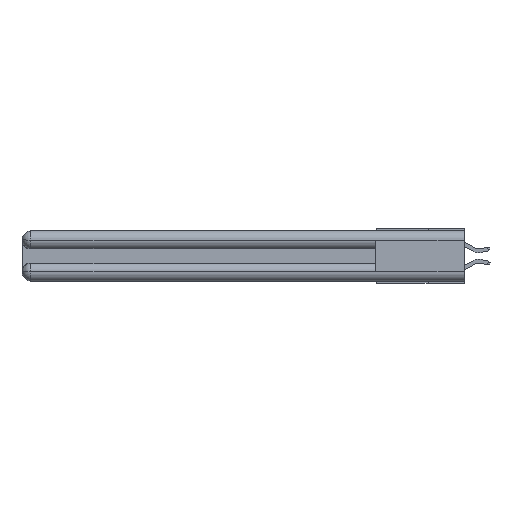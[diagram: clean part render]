
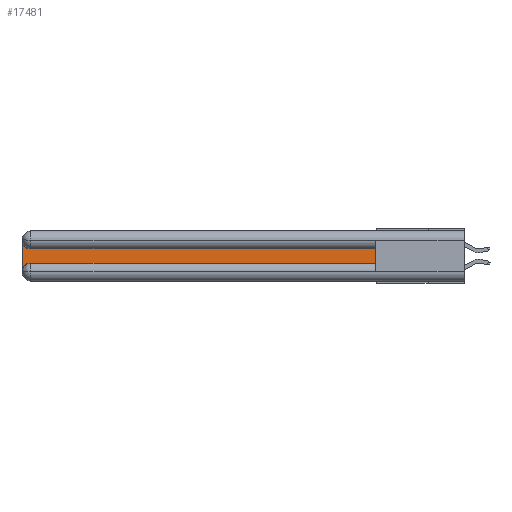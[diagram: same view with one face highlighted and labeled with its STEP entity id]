
A CAD part, left-side view. The second image highlights one B-rep face of the part: STEP entity #17481.
In plain terms, the highlighted planar face has unit normal (-1, 0, 0).
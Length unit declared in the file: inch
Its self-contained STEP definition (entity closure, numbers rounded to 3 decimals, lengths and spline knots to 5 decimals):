
#109 = AXIS2_PLACEMENT_3D ( 'NONE', #12864, #20478, #27432 ) ;
#374 = EDGE_CURVE ( 'NONE', #18083, #17569, #11368, .T. ) ;
#1002 = EDGE_LOOP ( 'NONE', ( #25631, #18869, #18796, #18351, #6841, #10107 ) ) ;
#1328 = CARTESIAN_POINT ( 'NONE',  ( 0.075, 3., -0.0625 ) ) ;
#2735 = EDGE_CURVE ( 'NONE', #17606, #11998, #6616, .T. ) ;
#4103 = DIRECTION ( 'NONE',  ( 0., 0., -1. ) ) ;
#4303 = LINE ( 'NONE', #16576, #23437 ) ;
#5975 = VERTEX_POINT ( 'NONE', #31462 ) ;
#6616 = LINE ( 'NONE', #9238, #14038 ) ;
#6841 = ORIENTED_EDGE ( 'NONE', *, *, #374, .T. ) ;
#8854 = DIRECTION ( 'NONE',  ( 0., 1., 0. ) ) ;
#8981 = EDGE_CURVE ( 'NONE', #17569, #5975, #31895, .T. ) ;
#9238 = CARTESIAN_POINT ( 'NONE',  ( 0.075, 3., -0.2175 ) ) ;
#10107 = ORIENTED_EDGE ( 'NONE', *, *, #8981, .T. ) ;
#11368 = LINE ( 'NONE', #29456, #12926 ) ;
#11998 = VERTEX_POINT ( 'NONE', #20435 ) ;
#12864 = CARTESIAN_POINT ( 'NONE',  ( 0.075, 2.94, -0.0625 ) ) ;
#12926 = VECTOR ( 'NONE', #17162, 39.37008 ) ;
#14038 = VECTOR ( 'NONE', #4103, 39.37008 ) ;
#15413 = DIRECTION ( 'NONE',  ( 0., 0., -1. ) ) ;
#16024 = AXIS2_PLACEMENT_3D ( 'NONE', #31465, #26398, #19001 ) ;
#16123 = CARTESIAN_POINT ( 'NONE',  ( 0.075, 2.94, -0.2175 ) ) ;
#16141 = VERTEX_POINT ( 'NONE', #28386 ) ;
#16576 = CARTESIAN_POINT ( 'NONE',  ( 0.075, 0.6, -0.1225 ) ) ;
#17162 = DIRECTION ( 'NONE',  ( 0., -1., 0. ) ) ;
#17481 = ADVANCED_FACE ( 'NONE', ( #19691 ), #20323, .F. ) ;
#17569 = VERTEX_POINT ( 'NONE', #18448 ) ;
#17606 = VERTEX_POINT ( 'NONE', #1328 ) ;
#18083 = VERTEX_POINT ( 'NONE', #16123 ) ;
#18351 = ORIENTED_EDGE ( 'NONE', *, *, #27183, .T. ) ;
#18448 = CARTESIAN_POINT ( 'NONE',  ( 0.075, 0.6, -0.2175 ) ) ;
#18796 = ORIENTED_EDGE ( 'NONE', *, *, #2735, .T. ) ;
#18869 = ORIENTED_EDGE ( 'NONE', *, *, #24911, .T. ) ;
#19001 = DIRECTION ( 'NONE',  ( 0., 0., -1. ) ) ;
#19691 = FACE_OUTER_BOUND ( 'NONE', #1002, .T. ) ;
#20323 = PLANE ( 'NONE',  #24620 ) ;
#20435 = CARTESIAN_POINT ( 'NONE',  ( 0.075, 3., -0.2775 ) ) ;
#20478 = DIRECTION ( 'NONE',  ( 1., 0., 0. ) ) ;
#20637 = CARTESIAN_POINT ( 'NONE',  ( 0.075, 3., -0.1225 ) ) ;
#21065 = VECTOR ( 'NONE', #25690, 39.37008 ) ;
#23437 = VECTOR ( 'NONE', #8854, 39.37008 ) ;
#24620 = AXIS2_PLACEMENT_3D ( 'NONE', #20637, #30327, #15413 ) ;
#24911 = EDGE_CURVE ( 'NONE', #16141, #17606, #26994, .T. ) ;
#25631 = ORIENTED_EDGE ( 'NONE', *, *, #25928, .T. ) ;
#25690 = DIRECTION ( 'NONE',  ( 0., 0., 1. ) ) ;
#25928 = EDGE_CURVE ( 'NONE', #5975, #16141, #4303, .T. ) ;
#26398 = DIRECTION ( 'NONE',  ( 1., 0., 0. ) ) ;
#26994 = CIRCLE ( 'NONE', #109, 0.06 ) ;
#27183 = EDGE_CURVE ( 'NONE', #11998, #18083, #30236, .T. ) ;
#27432 = DIRECTION ( 'NONE',  ( 0., 0., -1. ) ) ;
#28386 = CARTESIAN_POINT ( 'NONE',  ( 0.075, 2.94, -0.1225 ) ) ;
#29456 = CARTESIAN_POINT ( 'NONE',  ( 0.075, 0.6, -0.2175 ) ) ;
#30236 = CIRCLE ( 'NONE', #16024, 0.06 ) ;
#30327 = DIRECTION ( 'NONE',  ( 1., 0., 0. ) ) ;
#30497 = CARTESIAN_POINT ( 'NONE',  ( 0.075, 0.6, -0.2175 ) ) ;
#31462 = CARTESIAN_POINT ( 'NONE',  ( 0.075, 0.6, -0.1225 ) ) ;
#31465 = CARTESIAN_POINT ( 'NONE',  ( 0.075, 2.94, -0.2775 ) ) ;
#31895 = LINE ( 'NONE', #30497, #21065 ) ;
